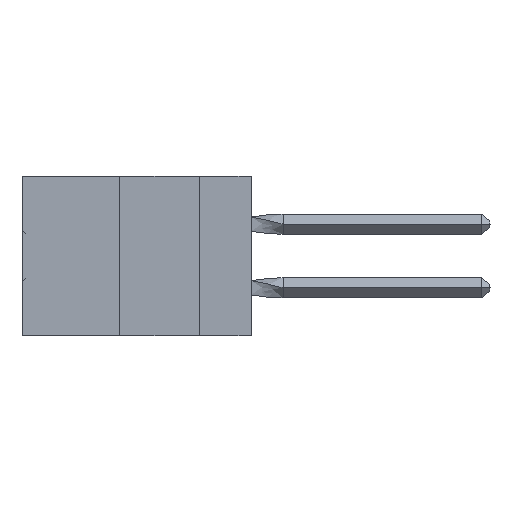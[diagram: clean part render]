
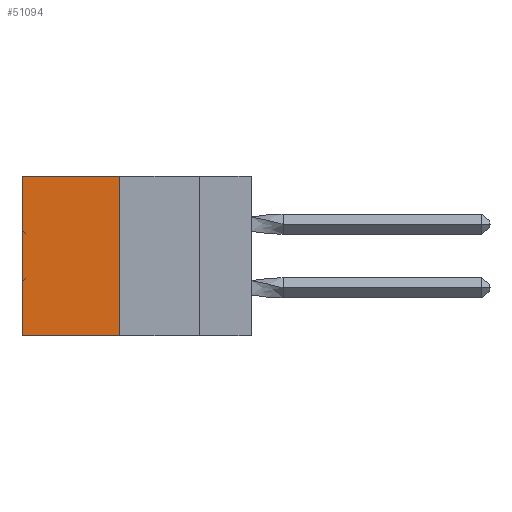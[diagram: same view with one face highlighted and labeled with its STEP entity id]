
A CAD part, left-side view. The second image highlights one B-rep face of the part: STEP entity #51094.
In plain terms, the highlighted planar face has unit normal (-1, 0, 0).
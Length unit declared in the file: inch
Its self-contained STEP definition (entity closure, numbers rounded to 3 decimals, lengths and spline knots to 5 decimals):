
#228 = VERTEX_POINT ( 'NONE', #54003 ) ;
#1756 = VECTOR ( 'NONE', #17832, 39.37008 ) ;
#2295 = LINE ( 'NONE', #8498, #28231 ) ;
#3113 = LINE ( 'NONE', #11806, #34729 ) ;
#4478 = DIRECTION ( 'NONE',  ( 1., 0., 0. ) ) ;
#6267 = LINE ( 'NONE', #15276, #40037 ) ;
#6393 = CARTESIAN_POINT ( 'NONE',  ( 0.305, 0.72, -0.5 ) ) ;
#8498 = CARTESIAN_POINT ( 'NONE',  ( 0.305, 0.413, -0.5 ) ) ;
#11806 = CARTESIAN_POINT ( 'NONE',  ( 0.305, 0.413, 0. ) ) ;
#13309 = EDGE_CURVE ( 'NONE', #41465, #47755, #3113, .T. ) ;
#13561 = DIRECTION ( 'NONE',  ( 0., 1., 0. ) ) ;
#14062 = LINE ( 'NONE', #54623, #1756 ) ;
#14948 = ORIENTED_EDGE ( 'NONE', *, *, #54210, .F. ) ;
#15276 = CARTESIAN_POINT ( 'NONE',  ( 0.305, 0.72, -0.5 ) ) ;
#17832 = DIRECTION ( 'NONE',  ( 0., 0., -1. ) ) ;
#20286 = DIRECTION ( 'NONE',  ( 0., 0., -1. ) ) ;
#22852 = FACE_OUTER_BOUND ( 'NONE', #41722, .T. ) ;
#23198 = CARTESIAN_POINT ( 'NONE',  ( 0.305, 0.413, -0.5 ) ) ;
#24922 = ORIENTED_EDGE ( 'NONE', *, *, #32730, .F. ) ;
#28231 = VECTOR ( 'NONE', #13561, 39.37008 ) ;
#29386 = ORIENTED_EDGE ( 'NONE', *, *, #13309, .T. ) ;
#32295 = CARTESIAN_POINT ( 'NONE',  ( 0.305, 0.413, 0. ) ) ;
#32730 = EDGE_CURVE ( 'NONE', #41465, #228, #14062, .T. ) ;
#34729 = VECTOR ( 'NONE', #34808, 39.37008 ) ;
#34808 = DIRECTION ( 'NONE',  ( 0., 1., 0. ) ) ;
#40037 = VECTOR ( 'NONE', #20286, 39.37008 ) ;
#40669 = VERTEX_POINT ( 'NONE', #6393 ) ;
#40887 = ORIENTED_EDGE ( 'NONE', *, *, #43569, .T. ) ;
#41247 = DIRECTION ( 'NONE',  ( 0., 0., -1. ) ) ;
#41465 = VERTEX_POINT ( 'NONE', #32295 ) ;
#41722 = EDGE_LOOP ( 'NONE', ( #40887, #14948, #24922, #29386 ) ) ;
#43569 = EDGE_CURVE ( 'NONE', #47755, #40669, #6267, .T. ) ;
#46934 = CARTESIAN_POINT ( 'NONE',  ( 0.305, 0.72, 0. ) ) ;
#47755 = VERTEX_POINT ( 'NONE', #46934 ) ;
#51094 = ADVANCED_FACE ( 'NONE', ( #22852 ), #55392, .F. ) ;
#52379 = AXIS2_PLACEMENT_3D ( 'NONE', #23198, #4478, #41247 ) ;
#54003 = CARTESIAN_POINT ( 'NONE',  ( 0.305, 0.413, -0.5 ) ) ;
#54210 = EDGE_CURVE ( 'NONE', #228, #40669, #2295, .T. ) ;
#54623 = CARTESIAN_POINT ( 'NONE',  ( 0.305, 0.413, -0.5 ) ) ;
#55392 = PLANE ( 'NONE',  #52379 ) ;
